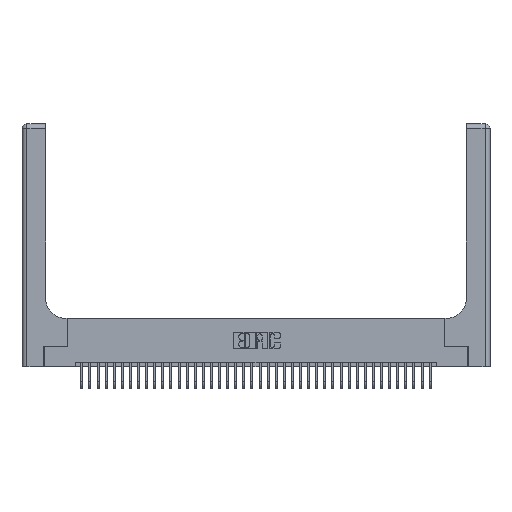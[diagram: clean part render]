
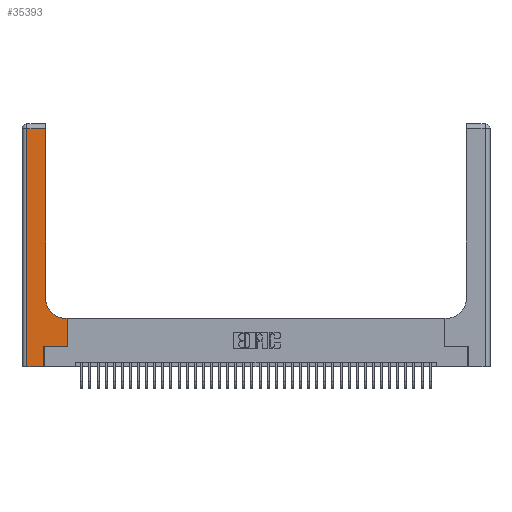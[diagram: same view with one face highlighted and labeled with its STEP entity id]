
A CAD part, top view. The second image highlights one B-rep face of the part: STEP entity #35393.
In plain terms, the highlighted planar face has unit normal (0, 0, 1).
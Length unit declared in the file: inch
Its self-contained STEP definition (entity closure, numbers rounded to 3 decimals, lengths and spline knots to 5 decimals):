
#2891 = ORIENTED_EDGE ( 'NONE', *, *, #38172, .T. ) ;
#2951 = VECTOR ( 'NONE', #9707, 39.37008 ) ;
#3423 = EDGE_CURVE ( 'NONE', #33402, #28260, #32299, .T. ) ;
#3634 = VERTEX_POINT ( 'NONE', #34533 ) ;
#4230 = DIRECTION ( 'NONE',  ( 0., 1., 0. ) ) ;
#4243 = ORIENTED_EDGE ( 'NONE', *, *, #35577, .T. ) ;
#6531 = VECTOR ( 'NONE', #4230, 39.37008 ) ;
#6841 = DIRECTION ( 'NONE',  ( 0., 1., 0. ) ) ;
#6981 = VERTEX_POINT ( 'NONE', #18981 ) ;
#7412 = LINE ( 'NONE', #28077, #17872 ) ;
#7634 = ORIENTED_EDGE ( 'NONE', *, *, #14152, .T. ) ;
#8331 = CARTESIAN_POINT ( 'NONE',  ( 0.2915, 0.6, 0.37 ) ) ;
#9020 = EDGE_CURVE ( 'NONE', #27423, #33402, #25340, .T. ) ;
#9707 = DIRECTION ( 'NONE',  ( 1., 0., 0. ) ) ;
#10808 = LINE ( 'NONE', #38720, #35088 ) ;
#11173 = EDGE_CURVE ( 'NONE', #3634, #21162, #24669, .T. ) ;
#11223 = EDGE_CURVE ( 'NONE', #21162, #6981, #21200, .T. ) ;
#11364 = ORIENTED_EDGE ( 'NONE', *, *, #3423, .T. ) ;
#11619 = ORIENTED_EDGE ( 'NONE', *, *, #26840, .T. ) ;
#12834 = DIRECTION ( 'NONE',  ( 0., 1., 0. ) ) ;
#12907 = VERTEX_POINT ( 'NONE', #37118 ) ;
#13003 = VECTOR ( 'NONE', #6841, 39.37008 ) ;
#13877 = CARTESIAN_POINT ( 'NONE',  ( 0.2915, 3., 0.37 ) ) ;
#14152 = EDGE_CURVE ( 'NONE', #37368, #12907, #10808, .T. ) ;
#14400 = PLANE ( 'NONE',  #23387 ) ;
#16357 = DIRECTION ( 'NONE',  ( -1., 0., 0. ) ) ;
#16587 = CARTESIAN_POINT ( 'NONE',  ( 0.269, 0., 0.37 ) ) ;
#17872 = VECTOR ( 'NONE', #12834, 39.37008 ) ;
#18003 = LINE ( 'NONE', #13877, #6531 ) ;
#18981 = CARTESIAN_POINT ( 'NONE',  ( 0.2915, 0.85, 0.37 ) ) ;
#19134 = CARTESIAN_POINT ( 'NONE',  ( 0., 0., 0.37 ) ) ;
#20298 = CARTESIAN_POINT ( 'NONE',  ( 0.06, 2.94, 0.37 ) ) ;
#21068 = VECTOR ( 'NONE', #16357, 39.37008 ) ;
#21162 = VERTEX_POINT ( 'NONE', #38317 ) ;
#21200 = CIRCLE ( 'NONE', #24661, 0.25 ) ;
#22828 = ORIENTED_EDGE ( 'NONE', *, *, #39525, .T. ) ;
#23336 = VECTOR ( 'NONE', #26577, 39.37008 ) ;
#23359 = CARTESIAN_POINT ( 'NONE',  ( 0.06, 3., 0.37 ) ) ;
#23387 = AXIS2_PLACEMENT_3D ( 'NONE', #36671, #36543, #27951 ) ;
#23828 = ORIENTED_EDGE ( 'NONE', *, *, #11223, .T. ) ;
#24661 = AXIS2_PLACEMENT_3D ( 'NONE', #39023, #29888, #34038 ) ;
#24669 = LINE ( 'NONE', #8331, #35515 ) ;
#25120 = DIRECTION ( 'NONE',  ( -1., 0., 0. ) ) ;
#25340 = LINE ( 'NONE', #23359, #23336 ) ;
#25365 = CARTESIAN_POINT ( 'NONE',  ( 0., 2.94, 0.37 ) ) ;
#26577 = DIRECTION ( 'NONE',  ( 0., -1., 0. ) ) ;
#26840 = EDGE_CURVE ( 'NONE', #6981, #35921, #18003, .T. ) ;
#27423 = VERTEX_POINT ( 'NONE', #20298 ) ;
#27951 = DIRECTION ( 'NONE',  ( -1., 0., 0. ) ) ;
#28020 = ORIENTED_EDGE ( 'NONE', *, *, #11173, .T. ) ;
#28077 = CARTESIAN_POINT ( 'NONE',  ( 0.5585, 0.25, 0.37 ) ) ;
#28260 = VERTEX_POINT ( 'NONE', #40721 ) ;
#28732 = CARTESIAN_POINT ( 'NONE',  ( 0.06, 0., 0.37 ) ) ;
#28785 = FACE_OUTER_BOUND ( 'NONE', #40149, .T. ) ;
#29721 = ORIENTED_EDGE ( 'NONE', *, *, #9020, .T. ) ;
#29888 = DIRECTION ( 'NONE',  ( 0., 0., -1. ) ) ;
#30552 = CARTESIAN_POINT ( 'NONE',  ( 0.2915, 2.94, 0.37 ) ) ;
#32299 = LINE ( 'NONE', #19134, #2951 ) ;
#32376 = LINE ( 'NONE', #16587, #13003 ) ;
#33402 = VERTEX_POINT ( 'NONE', #28732 ) ;
#34038 = DIRECTION ( 'NONE',  ( 1., 0., 0. ) ) ;
#34533 = CARTESIAN_POINT ( 'NONE',  ( 0.5585, 0.6, 0.37 ) ) ;
#35088 = VECTOR ( 'NONE', #39010, 39.37008 ) ;
#35393 = ADVANCED_FACE ( 'NONE', ( #28785 ), #14400, .F. ) ;
#35515 = VECTOR ( 'NONE', #25120, 39.37008 ) ;
#35577 = EDGE_CURVE ( 'NONE', #12907, #3634, #7412, .T. ) ;
#35921 = VERTEX_POINT ( 'NONE', #30552 ) ;
#36543 = DIRECTION ( 'NONE',  ( 0., 0., -1. ) ) ;
#36671 = CARTESIAN_POINT ( 'NONE',  ( 0., 3., 0.37 ) ) ;
#36933 = LINE ( 'NONE', #25365, #21068 ) ;
#37118 = CARTESIAN_POINT ( 'NONE',  ( 0.5585, 0.25, 0.37 ) ) ;
#37368 = VERTEX_POINT ( 'NONE', #37611 ) ;
#37611 = CARTESIAN_POINT ( 'NONE',  ( 0.269, 0.25, 0.37 ) ) ;
#38172 = EDGE_CURVE ( 'NONE', #28260, #37368, #32376, .T. ) ;
#38317 = CARTESIAN_POINT ( 'NONE',  ( 0.5415, 0.6, 0.37 ) ) ;
#38720 = CARTESIAN_POINT ( 'NONE',  ( 0.269, 0.25, 0.37 ) ) ;
#39010 = DIRECTION ( 'NONE',  ( 1., 0., 0. ) ) ;
#39023 = CARTESIAN_POINT ( 'NONE',  ( 0.5415, 0.85, 0.37 ) ) ;
#39525 = EDGE_CURVE ( 'NONE', #35921, #27423, #36933, .T. ) ;
#40149 = EDGE_LOOP ( 'NONE', ( #11619, #22828, #29721, #11364, #2891, #7634, #4243, #28020, #23828 ) ) ;
#40721 = CARTESIAN_POINT ( 'NONE',  ( 0.269, 0., 0.37 ) ) ;
